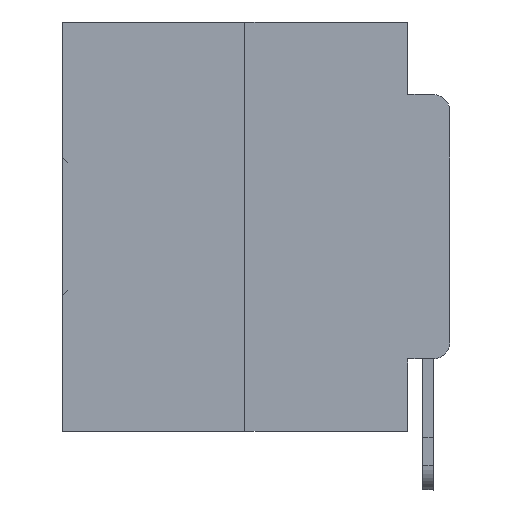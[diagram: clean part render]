
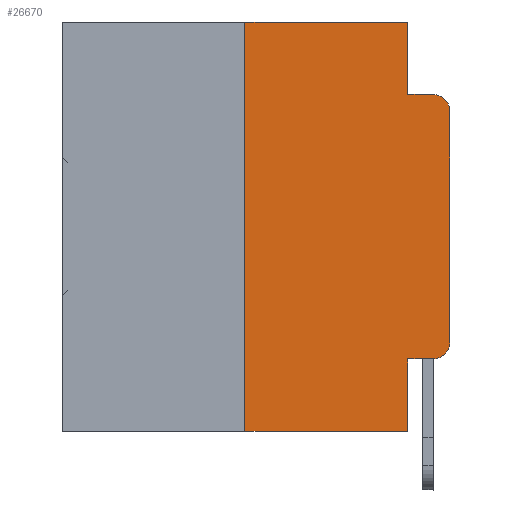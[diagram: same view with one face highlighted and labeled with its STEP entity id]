
A CAD part, left-side view. The second image highlights one B-rep face of the part: STEP entity #26670.
In plain terms, the highlighted planar face has unit normal (-1, 0, 0).
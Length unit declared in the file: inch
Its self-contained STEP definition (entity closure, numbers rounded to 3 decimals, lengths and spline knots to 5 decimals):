
#1372 = EDGE_LOOP ( 'NONE', ( #31830, #33197, #22721, #28479, #30566, #20227, #10968, #14671, #10502, #9166 ) ) ;
#1554 = CARTESIAN_POINT ( 'NONE',  ( 0., 0.02, -0.3915 ) ) ;
#1569 = CARTESIAN_POINT ( 'NONE',  ( 0., 0.473, -0.5 ) ) ;
#1835 = EDGE_CURVE ( 'NONE', #13917, #21191, #31851, .T. ) ;
#2207 = CARTESIAN_POINT ( 'NONE',  ( 0., 0.051, -0.4115 ) ) ;
#2646 = FACE_OUTER_BOUND ( 'NONE', #1372, .T. ) ;
#2819 = LINE ( 'NONE', #13096, #26320 ) ;
#2837 = VERTEX_POINT ( 'NONE', #8862 ) ;
#3241 = CARTESIAN_POINT ( 'NONE',  ( 0., 0., -0.1085 ) ) ;
#4335 = DIRECTION ( 'NONE',  ( 0., -1., 0. ) ) ;
#5434 = DIRECTION ( 'NONE',  ( 0., 0., -1. ) ) ;
#6264 = EDGE_CURVE ( 'NONE', #17189, #2837, #25203, .T. ) ;
#6813 = VERTEX_POINT ( 'NONE', #23643 ) ;
#8203 = AXIS2_PLACEMENT_3D ( 'NONE', #28995, #13673, #5434 ) ;
#8319 = VECTOR ( 'NONE', #30573, 39.37008 ) ;
#8834 = VECTOR ( 'NONE', #9480, 39.37008 ) ;
#8862 = CARTESIAN_POINT ( 'NONE',  ( 0., 0.02, -0.4115 ) ) ;
#9166 = ORIENTED_EDGE ( 'NONE', *, *, #17223, .T. ) ;
#9175 = EDGE_CURVE ( 'NONE', #21270, #21191, #32805, .T. ) ;
#9480 = DIRECTION ( 'NONE',  ( 0., -1., 0. ) ) ;
#10021 = CARTESIAN_POINT ( 'NONE',  ( 0., 0.051, -0.5 ) ) ;
#10385 = CARTESIAN_POINT ( 'NONE',  ( 0., 0.473, 0. ) ) ;
#10502 = ORIENTED_EDGE ( 'NONE', *, *, #6264, .T. ) ;
#10756 = EDGE_CURVE ( 'NONE', #20445, #28964, #25470, .T. ) ;
#10882 = EDGE_CURVE ( 'NONE', #11747, #13917, #33164, .T. ) ;
#10968 = ORIENTED_EDGE ( 'NONE', *, *, #28693, .T. ) ;
#11177 = CARTESIAN_POINT ( 'NONE',  ( 0., 0.051, 0. ) ) ;
#11747 = VERTEX_POINT ( 'NONE', #29298 ) ;
#11841 = DIRECTION ( 'NONE',  ( -1., 0., 0. ) ) ;
#12424 = CARTESIAN_POINT ( 'NONE',  ( 0., 0.25, -0.5 ) ) ;
#12517 = CARTESIAN_POINT ( 'NONE',  ( 0., 0.25, 0. ) ) ;
#12936 = DIRECTION ( 'NONE',  ( 0., -1., 0. ) ) ;
#13096 = CARTESIAN_POINT ( 'NONE',  ( 0., 0.473, 0. ) ) ;
#13269 = DIRECTION ( 'NONE',  ( 1., 0., 0. ) ) ;
#13673 = DIRECTION ( 'NONE',  ( -1., 0., 0. ) ) ;
#13917 = VERTEX_POINT ( 'NONE', #3241 ) ;
#14556 = CARTESIAN_POINT ( 'NONE',  ( 0., 0.051, 0. ) ) ;
#14671 = ORIENTED_EDGE ( 'NONE', *, *, #16974, .F. ) ;
#14722 = DIRECTION ( 'NONE',  ( 0., 0., 1. ) ) ;
#15867 = AXIS2_PLACEMENT_3D ( 'NONE', #1554, #11841, #17071 ) ;
#16375 = CIRCLE ( 'NONE', #15867, 0.02 ) ;
#16760 = VECTOR ( 'NONE', #32727, 39.37008 ) ;
#16974 = EDGE_CURVE ( 'NONE', #17189, #25545, #31717, .T. ) ;
#16990 = CARTESIAN_POINT ( 'NONE',  ( 0., 0.051, -0.0885 ) ) ;
#17071 = DIRECTION ( 'NONE',  ( 0., 0., -1. ) ) ;
#17189 = VERTEX_POINT ( 'NONE', #2207 ) ;
#17223 = EDGE_CURVE ( 'NONE', #2837, #11747, #16375, .T. ) ;
#18149 = PLANE ( 'NONE',  #32303 ) ;
#19030 = VECTOR ( 'NONE', #24459, 39.37008 ) ;
#19087 = CARTESIAN_POINT ( 'NONE',  ( 0., 0.02, -0.0885 ) ) ;
#19759 = LINE ( 'NONE', #14556, #16760 ) ;
#20028 = CARTESIAN_POINT ( 'NONE',  ( 0., 0., 0. ) ) ;
#20227 = ORIENTED_EDGE ( 'NONE', *, *, #10756, .F. ) ;
#20445 = VERTEX_POINT ( 'NONE', #12424 ) ;
#21009 = DIRECTION ( 'NONE',  ( 0., 0., -1. ) ) ;
#21191 = VERTEX_POINT ( 'NONE', #19087 ) ;
#21270 = VERTEX_POINT ( 'NONE', #24961 ) ;
#22468 = VECTOR ( 'NONE', #14722, 39.37008 ) ;
#22676 = CARTESIAN_POINT ( 'NONE',  ( 0., 0.051, -0.4115 ) ) ;
#22721 = ORIENTED_EDGE ( 'NONE', *, *, #9175, .F. ) ;
#23643 = CARTESIAN_POINT ( 'NONE',  ( 0., 0.051, 0. ) ) ;
#23728 = EDGE_CURVE ( 'NONE', #28964, #6813, #2819, .T. ) ;
#24459 = DIRECTION ( 'NONE',  ( 0., 0., -1. ) ) ;
#24961 = CARTESIAN_POINT ( 'NONE',  ( 0., 0.051, -0.0885 ) ) ;
#25203 = LINE ( 'NONE', #22676, #8319 ) ;
#25470 = LINE ( 'NONE', #12517, #22468 ) ;
#25545 = VERTEX_POINT ( 'NONE', #10021 ) ;
#25571 = DIRECTION ( 'NONE',  ( 0., 0., 1. ) ) ;
#26320 = VECTOR ( 'NONE', #12936, 39.37008 ) ;
#26670 = ADVANCED_FACE ( 'NONE', ( #2646 ), #18149, .F. ) ;
#27383 = EDGE_CURVE ( 'NONE', #6813, #21270, #19759, .T. ) ;
#27732 = VECTOR ( 'NONE', #4335, 39.37008 ) ;
#28479 = ORIENTED_EDGE ( 'NONE', *, *, #27383, .F. ) ;
#28693 = EDGE_CURVE ( 'NONE', #20445, #25545, #29855, .T. ) ;
#28782 = VECTOR ( 'NONE', #25571, 39.37008 ) ;
#28964 = VERTEX_POINT ( 'NONE', #31696 ) ;
#28995 = CARTESIAN_POINT ( 'NONE',  ( 0., 0.02, -0.1085 ) ) ;
#29298 = CARTESIAN_POINT ( 'NONE',  ( 0., 0., -0.3915 ) ) ;
#29855 = LINE ( 'NONE', #1569, #8834 ) ;
#30566 = ORIENTED_EDGE ( 'NONE', *, *, #23728, .F. ) ;
#30573 = DIRECTION ( 'NONE',  ( 0., -1., 0. ) ) ;
#31696 = CARTESIAN_POINT ( 'NONE',  ( 0., 0.25, 0. ) ) ;
#31717 = LINE ( 'NONE', #11177, #19030 ) ;
#31830 = ORIENTED_EDGE ( 'NONE', *, *, #10882, .T. ) ;
#31851 = CIRCLE ( 'NONE', #8203, 0.02 ) ;
#32303 = AXIS2_PLACEMENT_3D ( 'NONE', #10385, #13269, #21009 ) ;
#32727 = DIRECTION ( 'NONE',  ( 0., 0., -1. ) ) ;
#32805 = LINE ( 'NONE', #16990, #27732 ) ;
#33164 = LINE ( 'NONE', #20028, #28782 ) ;
#33197 = ORIENTED_EDGE ( 'NONE', *, *, #1835, .T. ) ;
